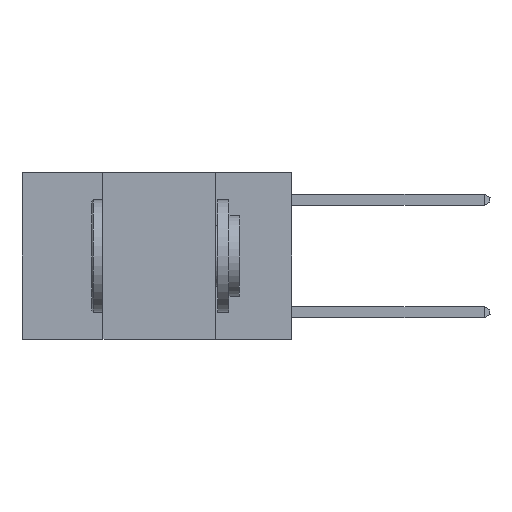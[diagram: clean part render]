
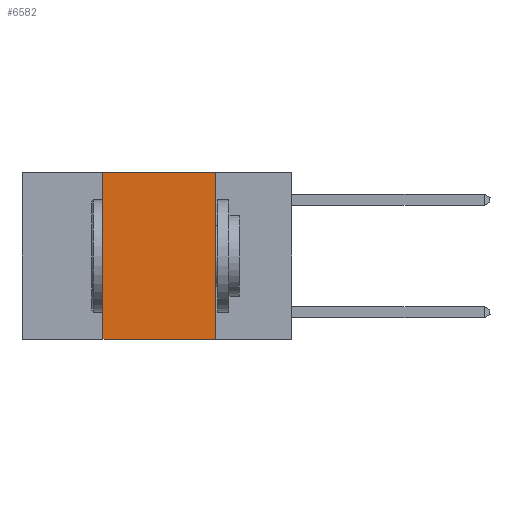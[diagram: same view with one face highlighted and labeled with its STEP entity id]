
A CAD part, left-side view. The second image highlights one B-rep face of the part: STEP entity #6582.
In plain terms, the highlighted planar face has unit normal (-1, 0, 0).
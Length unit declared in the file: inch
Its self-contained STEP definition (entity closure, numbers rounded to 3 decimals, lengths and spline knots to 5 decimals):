
#329 = CARTESIAN_POINT ( 'NONE',  ( 0., 0.6, 0. ) ) ;
#347 = CARTESIAN_POINT ( 'NONE',  ( 0., 0.17, 0. ) ) ;
#561 = DIRECTION ( 'NONE',  ( 1., 0., 0. ) ) ;
#565 = VERTEX_POINT ( 'NONE', #11559 ) ;
#641 = AXIS2_PLACEMENT_3D ( 'NONE', #10053, #561, #4782 ) ;
#838 = EDGE_CURVE ( 'NONE', #13412, #565, #4619, .T. ) ;
#858 = ORIENTED_EDGE ( 'NONE', *, *, #838, .F. ) ;
#1025 = LINE ( 'NONE', #11755, #1394 ) ;
#1110 = EDGE_CURVE ( 'NONE', #565, #11643, #12187, .T. ) ;
#1127 = VECTOR ( 'NONE', #4787, 39.37008 ) ;
#1394 = VECTOR ( 'NONE', #9733, 39.37008 ) ;
#1929 = CARTESIAN_POINT ( 'NONE',  ( 0., 0.17, -0.37 ) ) ;
#2745 = ORIENTED_EDGE ( 'NONE', *, *, #1110, .F. ) ;
#4419 = CARTESIAN_POINT ( 'NONE',  ( 0., 0.42, 0. ) ) ;
#4530 = ORIENTED_EDGE ( 'NONE', *, *, #12599, .T. ) ;
#4619 = LINE ( 'NONE', #329, #6007 ) ;
#4782 = DIRECTION ( 'NONE',  ( 0., 0., -1. ) ) ;
#4787 = DIRECTION ( 'NONE',  ( 0., 0., -1. ) ) ;
#4854 = CARTESIAN_POINT ( 'NONE',  ( 0., 0.42, -0.37 ) ) ;
#5731 = LINE ( 'NONE', #10192, #13158 ) ;
#5899 = EDGE_LOOP ( 'NONE', ( #2745, #858, #10236, #4530 ) ) ;
#6007 = VECTOR ( 'NONE', #12902, 39.37008 ) ;
#6073 = EDGE_CURVE ( 'NONE', #8408, #13412, #5731, .T. ) ;
#6139 = DIRECTION ( 'NONE',  ( 0., 0., 1. ) ) ;
#6582 = ADVANCED_FACE ( 'NONE', ( #8117 ), #12307, .F. ) ;
#8117 = FACE_OUTER_BOUND ( 'NONE', #5899, .T. ) ;
#8408 = VERTEX_POINT ( 'NONE', #4854 ) ;
#9733 = DIRECTION ( 'NONE',  ( 0., -1., 0. ) ) ;
#10053 = CARTESIAN_POINT ( 'NONE',  ( 0., 0.6, 0. ) ) ;
#10192 = CARTESIAN_POINT ( 'NONE',  ( 0., 0.42, 0. ) ) ;
#10236 = ORIENTED_EDGE ( 'NONE', *, *, #6073, .F. ) ;
#11559 = CARTESIAN_POINT ( 'NONE',  ( 0., 0.17, 0. ) ) ;
#11643 = VERTEX_POINT ( 'NONE', #1929 ) ;
#11755 = CARTESIAN_POINT ( 'NONE',  ( 0., 0.6, -0.37 ) ) ;
#12187 = LINE ( 'NONE', #347, #1127 ) ;
#12307 = PLANE ( 'NONE',  #641 ) ;
#12599 = EDGE_CURVE ( 'NONE', #8408, #11643, #1025, .T. ) ;
#12902 = DIRECTION ( 'NONE',  ( 0., -1., 0. ) ) ;
#13158 = VECTOR ( 'NONE', #6139, 39.37008 ) ;
#13412 = VERTEX_POINT ( 'NONE', #4419 ) ;
